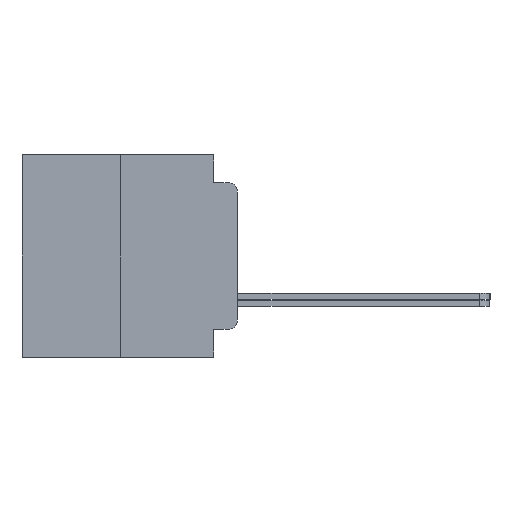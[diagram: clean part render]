
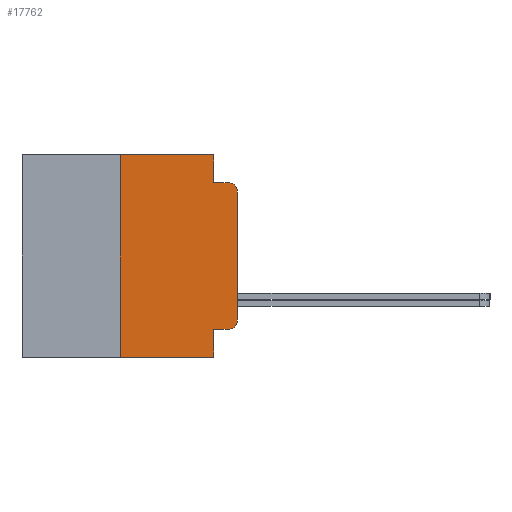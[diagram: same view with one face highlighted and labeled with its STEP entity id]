
A CAD part, left-side view. The second image highlights one B-rep face of the part: STEP entity #17762.
In plain terms, the highlighted planar face has unit normal (-1, 0, 0).
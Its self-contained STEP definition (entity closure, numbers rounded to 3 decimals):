
#166 = VERTEX_POINT ( 'NONE', #15703 ) ;
#882 = CARTESIAN_POINT ( 'NONE',  ( -75.603, 0.508, 3.975 ) ) ;
#954 = CARTESIAN_POINT ( 'NONE',  ( -75.603, 0., 3.467 ) ) ;
#1038 = ORIENTED_EDGE ( 'NONE', *, *, #23745, .F. ) ;
#1279 = ORIENTED_EDGE ( 'NONE', *, *, #1762, .F. ) ;
#1282 = VERTEX_POINT ( 'NONE', #2553 ) ;
#1762 = EDGE_CURVE ( 'NONE', #4991, #16304, #5512, .T. ) ;
#1787 = LINE ( 'NONE', #13234, #13389 ) ;
#2086 = CARTESIAN_POINT ( 'NONE',  ( -75.603, 0.508, -3.467 ) ) ;
#2236 = CARTESIAN_POINT ( 'NONE',  ( -75.603, 1.295, 3.975 ) ) ;
#2553 = CARTESIAN_POINT ( 'NONE',  ( -75.603, 6.35, -5.486 ) ) ;
#3415 = PLANE ( 'NONE',  #23276 ) ;
#3782 = VECTOR ( 'NONE', #13212, 1000. ) ;
#4127 = AXIS2_PLACEMENT_3D ( 'NONE', #6610, #23356, #12879 ) ;
#4991 = VERTEX_POINT ( 'NONE', #2236 ) ;
#5512 = LINE ( 'NONE', #22984, #7497 ) ;
#5649 = CARTESIAN_POINT ( 'NONE',  ( -75.603, 11.684, 5.486 ) ) ;
#5693 = EDGE_CURVE ( 'NONE', #19194, #4991, #24567, .T. ) ;
#5759 = VECTOR ( 'NONE', #14866, 1000. ) ;
#6143 = ORIENTED_EDGE ( 'NONE', *, *, #24306, .F. ) ;
#6610 = CARTESIAN_POINT ( 'NONE',  ( -75.603, 0.508, 3.467 ) ) ;
#6722 = EDGE_CURVE ( 'NONE', #12470, #13877, #16923, .T. ) ;
#7114 = ORIENTED_EDGE ( 'NONE', *, *, #14224, .T. ) ;
#7497 = VECTOR ( 'NONE', #16407, 1000. ) ;
#8493 = DIRECTION ( 'NONE',  ( 0., 0., -1. ) ) ;
#8669 = VERTEX_POINT ( 'NONE', #22121 ) ;
#8975 = CARTESIAN_POINT ( 'NONE',  ( -75.603, 1.295, -3.975 ) ) ;
#9074 = LINE ( 'NONE', #17075, #5759 ) ;
#9244 = CARTESIAN_POINT ( 'NONE',  ( -75.603, 1.295, 0. ) ) ;
#9338 = DIRECTION ( 'NONE',  ( 0., 0., -1. ) ) ;
#10698 = DIRECTION ( 'NONE',  ( 0., 0., 1. ) ) ;
#11507 = EDGE_CURVE ( 'NONE', #14414, #16304, #23536, .T. ) ;
#12068 = VERTEX_POINT ( 'NONE', #16859 ) ;
#12153 = ORIENTED_EDGE ( 'NONE', *, *, #15778, .T. ) ;
#12470 = VERTEX_POINT ( 'NONE', #21816 ) ;
#12499 = VECTOR ( 'NONE', #22375, 1000. ) ;
#12879 = DIRECTION ( 'NONE',  ( 0., 0., -1. ) ) ;
#13212 = DIRECTION ( 'NONE',  ( 0., 0., -1. ) ) ;
#13234 = CARTESIAN_POINT ( 'NONE',  ( -75.603, 6.35, -5.486 ) ) ;
#13389 = VECTOR ( 'NONE', #15476, 1000. ) ;
#13722 = DIRECTION ( 'NONE',  ( 0., -1., 0. ) ) ;
#13877 = VERTEX_POINT ( 'NONE', #24399 ) ;
#14031 = CARTESIAN_POINT ( 'NONE',  ( -75.603, 11.684, -5.486 ) ) ;
#14224 = EDGE_CURVE ( 'NONE', #13877, #8669, #20542, .T. ) ;
#14414 = VERTEX_POINT ( 'NONE', #954 ) ;
#14690 = ORIENTED_EDGE ( 'NONE', *, *, #6722, .T. ) ;
#14866 = DIRECTION ( 'NONE',  ( 0., -1., 0. ) ) ;
#15476 = DIRECTION ( 'NONE',  ( 0., 0., 1. ) ) ;
#15598 = VECTOR ( 'NONE', #13722, 1000. ) ;
#15668 = LINE ( 'NONE', #21454, #26302 ) ;
#15703 = CARTESIAN_POINT ( 'NONE',  ( -75.603, 1.295, -5.486 ) ) ;
#15778 = EDGE_CURVE ( 'NONE', #1282, #166, #15833, .T. ) ;
#15833 = LINE ( 'NONE', #14031, #12499 ) ;
#16076 = CARTESIAN_POINT ( 'NONE',  ( -75.603, 1.295, 5.486 ) ) ;
#16304 = VERTEX_POINT ( 'NONE', #882 ) ;
#16407 = DIRECTION ( 'NONE',  ( 0., -1., 0. ) ) ;
#16859 = CARTESIAN_POINT ( 'NONE',  ( -75.603, 6.35, 5.486 ) ) ;
#16923 = LINE ( 'NONE', #8975, #15598 ) ;
#16946 = EDGE_CURVE ( 'NONE', #1282, #12068, #1787, .T. ) ;
#17075 = CARTESIAN_POINT ( 'NONE',  ( -75.603, 11.684, 5.486 ) ) ;
#17762 = ADVANCED_FACE ( 'NONE', ( #26338 ), #3415, .F. ) ;
#17944 = ORIENTED_EDGE ( 'NONE', *, *, #20126, .T. ) ;
#19075 = DIRECTION ( 'NONE',  ( -1., 0., 0. ) ) ;
#19194 = VERTEX_POINT ( 'NONE', #16076 ) ;
#20054 = ORIENTED_EDGE ( 'NONE', *, *, #11507, .T. ) ;
#20126 = EDGE_CURVE ( 'NONE', #8669, #14414, #15668, .T. ) ;
#20542 = CIRCLE ( 'NONE', #26315, 0.508 ) ;
#20679 = DIRECTION ( 'NONE',  ( 1., 0., 0. ) ) ;
#20750 = EDGE_LOOP ( 'NONE', ( #14690, #7114, #17944, #20054, #1279, #23947, #6143, #21937, #12153, #1038 ) ) ;
#21341 = CARTESIAN_POINT ( 'NONE',  ( -75.603, 1.295, 0. ) ) ;
#21454 = CARTESIAN_POINT ( 'NONE',  ( -75.603, 0., 5.486 ) ) ;
#21816 = CARTESIAN_POINT ( 'NONE',  ( -75.603, 1.295, -3.975 ) ) ;
#21937 = ORIENTED_EDGE ( 'NONE', *, *, #16946, .F. ) ;
#22121 = CARTESIAN_POINT ( 'NONE',  ( -75.603, 0., -3.467 ) ) ;
#22375 = DIRECTION ( 'NONE',  ( 0., -1., 0. ) ) ;
#22984 = CARTESIAN_POINT ( 'NONE',  ( -75.603, 1.295, 3.975 ) ) ;
#23276 = AXIS2_PLACEMENT_3D ( 'NONE', #5649, #20679, #26770 ) ;
#23356 = DIRECTION ( 'NONE',  ( -1., 0., 0. ) ) ;
#23536 = CIRCLE ( 'NONE', #4127, 0.508 ) ;
#23745 = EDGE_CURVE ( 'NONE', #12470, #166, #24068, .T. ) ;
#23947 = ORIENTED_EDGE ( 'NONE', *, *, #5693, .F. ) ;
#24068 = LINE ( 'NONE', #21341, #3782 ) ;
#24306 = EDGE_CURVE ( 'NONE', #12068, #19194, #9074, .T. ) ;
#24399 = CARTESIAN_POINT ( 'NONE',  ( -75.603, 0.508, -3.975 ) ) ;
#24567 = LINE ( 'NONE', #9244, #26585 ) ;
#26302 = VECTOR ( 'NONE', #10698, 1000. ) ;
#26315 = AXIS2_PLACEMENT_3D ( 'NONE', #2086, #19075, #8493 ) ;
#26338 = FACE_OUTER_BOUND ( 'NONE', #20750, .T. ) ;
#26585 = VECTOR ( 'NONE', #9338, 1000. ) ;
#26770 = DIRECTION ( 'NONE',  ( 0., 0., -1. ) ) ;
